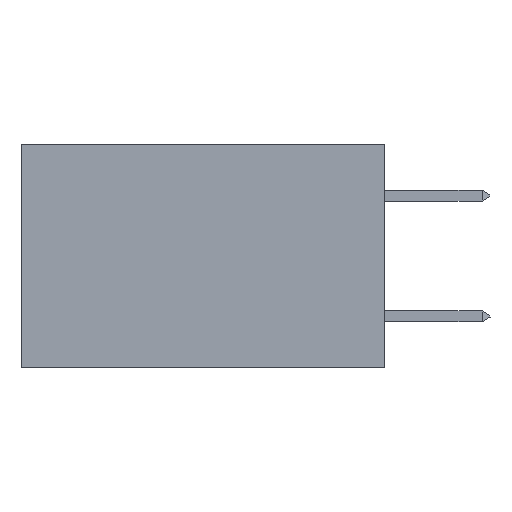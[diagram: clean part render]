
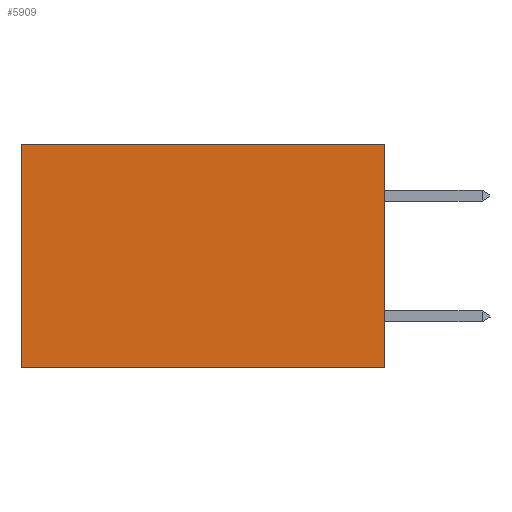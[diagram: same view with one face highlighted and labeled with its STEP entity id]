
A CAD part, left-side view. The second image highlights one B-rep face of the part: STEP entity #5909.
In plain terms, the highlighted planar face has unit normal (-1, 0, 0).
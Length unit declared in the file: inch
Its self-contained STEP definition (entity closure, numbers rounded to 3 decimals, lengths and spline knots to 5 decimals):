
#22 = DIRECTION ( 'NONE',  ( 0., 0., -1. ) ) ;
#621 = CARTESIAN_POINT ( 'NONE',  ( 0.2875, 0.6, 0. ) ) ;
#1198 = EDGE_LOOP ( 'NONE', ( #5196, #14090, #12670, #2261 ) ) ;
#1710 = VECTOR ( 'NONE', #10904, 39.37008 ) ;
#2206 = EDGE_CURVE ( 'NONE', #7784, #15028, #8915, .T. ) ;
#2261 = ORIENTED_EDGE ( 'NONE', *, *, #7243, .T. ) ;
#2362 = EDGE_CURVE ( 'NONE', #5572, #12308, #10379, .T. ) ;
#3473 = DIRECTION ( 'NONE',  ( 1., 0., 0. ) ) ;
#3566 = CARTESIAN_POINT ( 'NONE',  ( 0.2875, 0., -0.37 ) ) ;
#3921 = VECTOR ( 'NONE', #11148, 39.37008 ) ;
#4160 = FACE_OUTER_BOUND ( 'NONE', #1198, .T. ) ;
#4338 = CARTESIAN_POINT ( 'NONE',  ( 0.2875, 0., -0.37 ) ) ;
#5021 = LINE ( 'NONE', #7524, #3921 ) ;
#5196 = ORIENTED_EDGE ( 'NONE', *, *, #2206, .T. ) ;
#5572 = VERTEX_POINT ( 'NONE', #14410 ) ;
#5742 = LINE ( 'NONE', #4338, #8687 ) ;
#5760 = VECTOR ( 'NONE', #9608, 39.37008 ) ;
#5766 = DIRECTION ( 'NONE',  ( 0., 1., 0. ) ) ;
#5909 = ADVANCED_FACE ( 'NONE', ( #4160 ), #10684, .F. ) ;
#6503 = CARTESIAN_POINT ( 'NONE',  ( 0.2875, 0.6, -0.37 ) ) ;
#7243 = EDGE_CURVE ( 'NONE', #5572, #7784, #5021, .T. ) ;
#7524 = CARTESIAN_POINT ( 'NONE',  ( 0.2875, 0., 0. ) ) ;
#7784 = VERTEX_POINT ( 'NONE', #621 ) ;
#8687 = VECTOR ( 'NONE', #5766, 39.37008 ) ;
#8915 = LINE ( 'NONE', #11156, #5760 ) ;
#9357 = CARTESIAN_POINT ( 'NONE',  ( 0.2875, 0., 0. ) ) ;
#9608 = DIRECTION ( 'NONE',  ( 0., 0., -1. ) ) ;
#9702 = CARTESIAN_POINT ( 'NONE',  ( 0.2875, 0., 0. ) ) ;
#10379 = LINE ( 'NONE', #9702, #1710 ) ;
#10684 = PLANE ( 'NONE',  #11067 ) ;
#10904 = DIRECTION ( 'NONE',  ( 0., 0., -1. ) ) ;
#11067 = AXIS2_PLACEMENT_3D ( 'NONE', #9357, #3473, #22 ) ;
#11148 = DIRECTION ( 'NONE',  ( 0., 1., 0. ) ) ;
#11156 = CARTESIAN_POINT ( 'NONE',  ( 0.2875, 0.6, 0. ) ) ;
#12308 = VERTEX_POINT ( 'NONE', #3566 ) ;
#12670 = ORIENTED_EDGE ( 'NONE', *, *, #2362, .F. ) ;
#14090 = ORIENTED_EDGE ( 'NONE', *, *, #14998, .F. ) ;
#14410 = CARTESIAN_POINT ( 'NONE',  ( 0.2875, 0., 0. ) ) ;
#14998 = EDGE_CURVE ( 'NONE', #12308, #15028, #5742, .T. ) ;
#15028 = VERTEX_POINT ( 'NONE', #6503 ) ;
